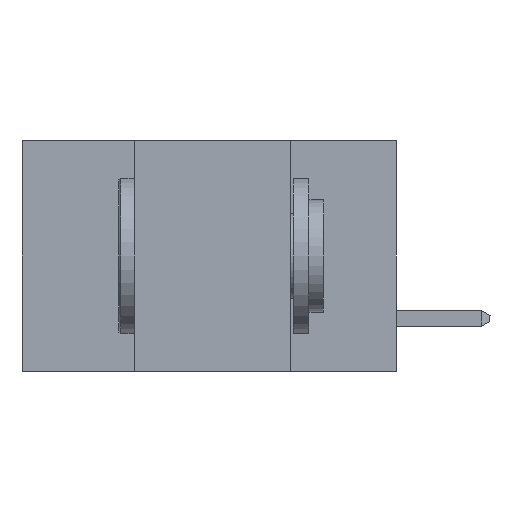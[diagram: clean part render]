
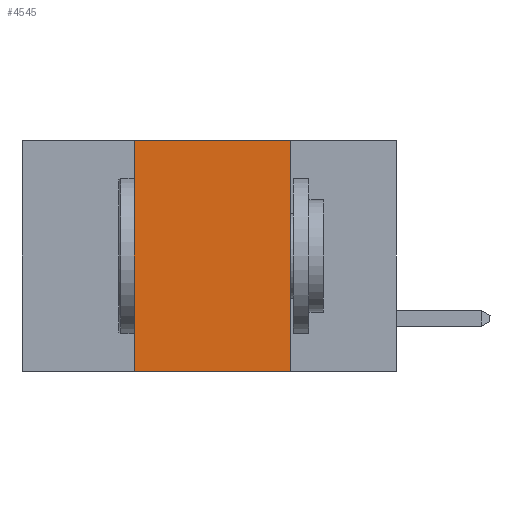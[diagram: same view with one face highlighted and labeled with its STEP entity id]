
A CAD part, left-side view. The second image highlights one B-rep face of the part: STEP entity #4545.
In plain terms, the highlighted planar face has unit normal (-1, 0, 0).
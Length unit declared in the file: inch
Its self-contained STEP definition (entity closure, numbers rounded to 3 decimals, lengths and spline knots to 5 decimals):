
#401 = ORIENTED_EDGE ( 'NONE', *, *, #1528, .F. ) ;
#958 = DIRECTION ( 'NONE',  ( 0., -1., 0. ) ) ;
#973 = VECTOR ( 'NONE', #958, 39.37008 ) ;
#1528 = EDGE_CURVE ( 'NONE', #3279, #9406, #9677, .T. ) ;
#1595 = DIRECTION ( 'NONE',  ( 0., 0., -1. ) ) ;
#1925 = DIRECTION ( 'NONE',  ( 0., -1., 0. ) ) ;
#2182 = VECTOR ( 'NONE', #1595, 39.37008 ) ;
#2358 = DIRECTION ( 'NONE',  ( 0., 0., -1. ) ) ;
#2405 = ORIENTED_EDGE ( 'NONE', *, *, #6307, .T. ) ;
#2830 = CARTESIAN_POINT ( 'NONE',  ( 0., 0.42, -0.37 ) ) ;
#2837 = AXIS2_PLACEMENT_3D ( 'NONE', #7797, #11327, #2358 ) ;
#3279 = VERTEX_POINT ( 'NONE', #7631 ) ;
#4259 = FACE_OUTER_BOUND ( 'NONE', #6961, .T. ) ;
#4545 = ADVANCED_FACE ( 'NONE', ( #4259 ), #11206, .F. ) ;
#5583 = DIRECTION ( 'NONE',  ( 0., 0., 1. ) ) ;
#6262 = LINE ( 'NONE', #10848, #9410 ) ;
#6307 = EDGE_CURVE ( 'NONE', #8816, #9406, #6262, .T. ) ;
#6550 = CARTESIAN_POINT ( 'NONE',  ( 0., 0.42, 0. ) ) ;
#6633 = LINE ( 'NONE', #2830, #9809 ) ;
#6961 = EDGE_LOOP ( 'NONE', ( #401, #9496, #11308, #2405 ) ) ;
#7191 = LINE ( 'NONE', #10676, #973 ) ;
#7631 = CARTESIAN_POINT ( 'NONE',  ( 0., 0.17, 0. ) ) ;
#7750 = VERTEX_POINT ( 'NONE', #6550 ) ;
#7797 = CARTESIAN_POINT ( 'NONE',  ( 0., 0.6, 0. ) ) ;
#7989 = EDGE_CURVE ( 'NONE', #7750, #3279, #7191, .T. ) ;
#8816 = VERTEX_POINT ( 'NONE', #8840 ) ;
#8840 = CARTESIAN_POINT ( 'NONE',  ( 0., 0.42, -0.37 ) ) ;
#9406 = VERTEX_POINT ( 'NONE', #10959 ) ;
#9410 = VECTOR ( 'NONE', #1925, 39.37008 ) ;
#9496 = ORIENTED_EDGE ( 'NONE', *, *, #7989, .F. ) ;
#9627 = CARTESIAN_POINT ( 'NONE',  ( 0., 0.17, -0.37 ) ) ;
#9677 = LINE ( 'NONE', #9627, #2182 ) ;
#9809 = VECTOR ( 'NONE', #5583, 39.37008 ) ;
#10437 = EDGE_CURVE ( 'NONE', #8816, #7750, #6633, .T. ) ;
#10676 = CARTESIAN_POINT ( 'NONE',  ( 0., 0.6, 0. ) ) ;
#10848 = CARTESIAN_POINT ( 'NONE',  ( 0., 0.6, -0.37 ) ) ;
#10959 = CARTESIAN_POINT ( 'NONE',  ( 0., 0.17, -0.37 ) ) ;
#11206 = PLANE ( 'NONE',  #2837 ) ;
#11308 = ORIENTED_EDGE ( 'NONE', *, *, #10437, .F. ) ;
#11327 = DIRECTION ( 'NONE',  ( 1., 0., 0. ) ) ;
